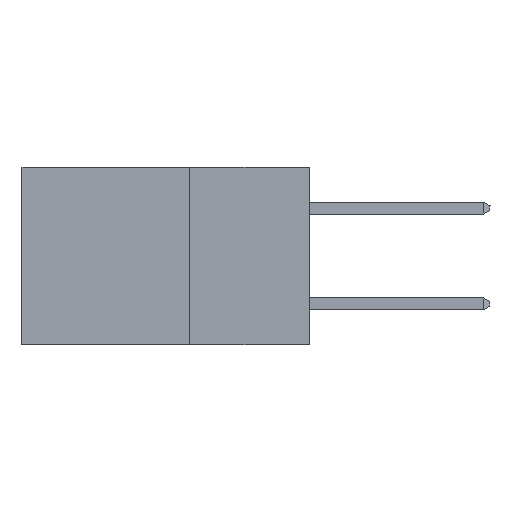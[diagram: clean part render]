
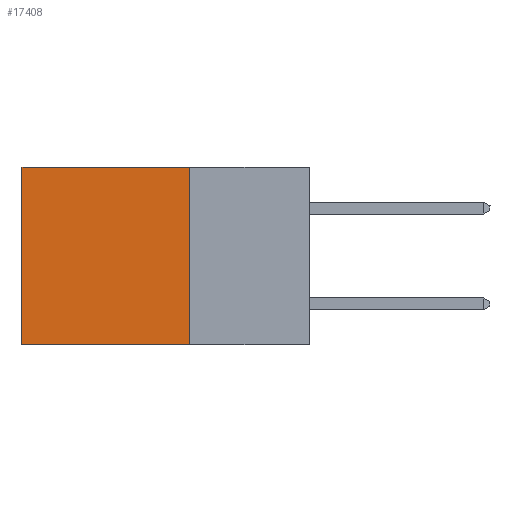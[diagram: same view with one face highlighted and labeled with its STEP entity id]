
A CAD part, left-side view. The second image highlights one B-rep face of the part: STEP entity #17408.
In plain terms, the highlighted planar face has unit normal (-1, 0, 0).
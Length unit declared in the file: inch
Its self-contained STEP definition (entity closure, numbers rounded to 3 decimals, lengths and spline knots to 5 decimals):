
#284 = EDGE_LOOP ( 'NONE', ( #1086, #10204, #9204, #6126 ) ) ;
#1086 = ORIENTED_EDGE ( 'NONE', *, *, #5540, .T. ) ;
#1311 = CARTESIAN_POINT ( 'NONE',  ( 0.2875, 0.25, 0. ) ) ;
#1357 = DIRECTION ( 'NONE',  ( 0., 0., -1. ) ) ;
#3375 = VERTEX_POINT ( 'NONE', #7150 ) ;
#4586 = EDGE_CURVE ( 'NONE', #15365, #5163, #8654, .T. ) ;
#5163 = VERTEX_POINT ( 'NONE', #7358 ) ;
#5280 = EDGE_CURVE ( 'NONE', #15365, #8083, #10770, .T. ) ;
#5540 = EDGE_CURVE ( 'NONE', #5163, #3375, #16143, .T. ) ;
#5696 = VECTOR ( 'NONE', #7190, 39.37008 ) ;
#5928 = CARTESIAN_POINT ( 'NONE',  ( 0.2875, 0.25, 0. ) ) ;
#6126 = ORIENTED_EDGE ( 'NONE', *, *, #4586, .T. ) ;
#7150 = CARTESIAN_POINT ( 'NONE',  ( 0.2875, 0.6, -0.37 ) ) ;
#7190 = DIRECTION ( 'NONE',  ( 0., 1., 0. ) ) ;
#7358 = CARTESIAN_POINT ( 'NONE',  ( 0.2875, 0.6, 0. ) ) ;
#7599 = LINE ( 'NONE', #12059, #16618 ) ;
#7976 = PLANE ( 'NONE',  #11963 ) ;
#8026 = CARTESIAN_POINT ( 'NONE',  ( 0.2875, 0.25, 0. ) ) ;
#8070 = FACE_OUTER_BOUND ( 'NONE', #284, .T. ) ;
#8083 = VERTEX_POINT ( 'NONE', #15696 ) ;
#8654 = LINE ( 'NONE', #1311, #5696 ) ;
#9204 = ORIENTED_EDGE ( 'NONE', *, *, #5280, .F. ) ;
#9596 = DIRECTION ( 'NONE',  ( 0., 0., -1. ) ) ;
#10204 = ORIENTED_EDGE ( 'NONE', *, *, #18581, .F. ) ;
#10770 = LINE ( 'NONE', #8026, #16769 ) ;
#10811 = DIRECTION ( 'NONE',  ( 0., 0., -1. ) ) ;
#11963 = AXIS2_PLACEMENT_3D ( 'NONE', #16594, #18134, #10811 ) ;
#12059 = CARTESIAN_POINT ( 'NONE',  ( 0.2875, 0.25, -0.37 ) ) ;
#13321 = CARTESIAN_POINT ( 'NONE',  ( 0.2875, 0.6, 0. ) ) ;
#13396 = DIRECTION ( 'NONE',  ( 0., 1., 0. ) ) ;
#15365 = VERTEX_POINT ( 'NONE', #5928 ) ;
#15696 = CARTESIAN_POINT ( 'NONE',  ( 0.2875, 0.25, -0.37 ) ) ;
#15786 = VECTOR ( 'NONE', #1357, 39.37008 ) ;
#16143 = LINE ( 'NONE', #13321, #15786 ) ;
#16594 = CARTESIAN_POINT ( 'NONE',  ( 0.2875, 0.25, 0. ) ) ;
#16618 = VECTOR ( 'NONE', #13396, 39.37008 ) ;
#16769 = VECTOR ( 'NONE', #9596, 39.37008 ) ;
#17408 = ADVANCED_FACE ( 'NONE', ( #8070 ), #7976, .F. ) ;
#18134 = DIRECTION ( 'NONE',  ( 1., 0., 0. ) ) ;
#18581 = EDGE_CURVE ( 'NONE', #8083, #3375, #7599, .T. ) ;
